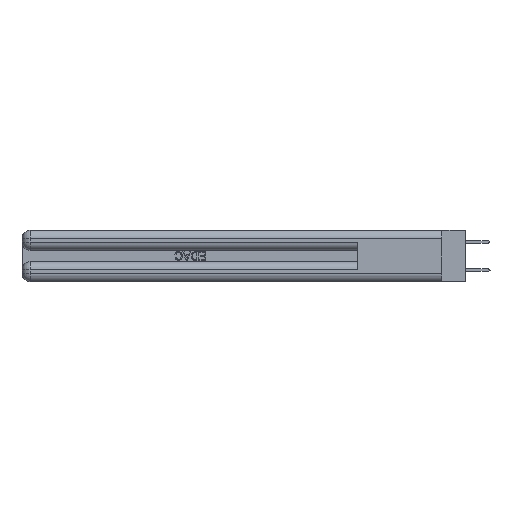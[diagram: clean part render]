
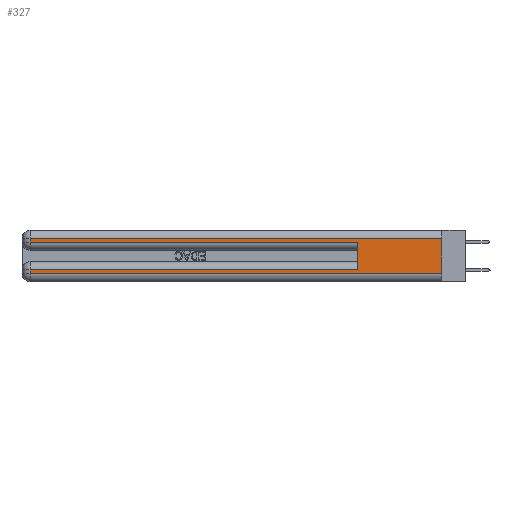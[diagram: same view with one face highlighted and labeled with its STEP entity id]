
A CAD part, left-side view. The second image highlights one B-rep face of the part: STEP entity #327.
In plain terms, the highlighted planar face has unit normal (-1, 0, 0).
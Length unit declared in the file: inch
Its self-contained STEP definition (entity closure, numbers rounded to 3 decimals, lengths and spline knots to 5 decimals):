
#327 = ADVANCED_FACE ( 'NONE', ( #8994 ), #20867, .F. ) ;
#1510 = LINE ( 'NONE', #37343, #40976 ) ;
#2214 = ORIENTED_EDGE ( 'NONE', *, *, #22925, .F. ) ;
#2718 = CARTESIAN_POINT ( 'NONE',  ( 0., 2.94, 0.37 ) ) ;
#3404 = ORIENTED_EDGE ( 'NONE', *, *, #18552, .T. ) ;
#4596 = DIRECTION ( 'NONE',  ( 0., -1., 0. ) ) ;
#6879 = DIRECTION ( 'NONE',  ( 0., 0., 1. ) ) ;
#6996 = ORIENTED_EDGE ( 'NONE', *, *, #29429, .T. ) ;
#7479 = VERTEX_POINT ( 'NONE', #31076 ) ;
#8994 = FACE_OUTER_BOUND ( 'NONE', #10043, .T. ) ;
#9367 = LINE ( 'NONE', #2718, #28560 ) ;
#9704 = CARTESIAN_POINT ( 'NONE',  ( 0., 0., 0.37 ) ) ;
#10043 = EDGE_LOOP ( 'NONE', ( #32769, #3404, #6996, #31560, #2214, #26198, #10621, #19074 ) ) ;
#10202 = DIRECTION ( 'NONE',  ( 0., 1., 0. ) ) ;
#10621 = ORIENTED_EDGE ( 'NONE', *, *, #47641, .T. ) ;
#10804 = VERTEX_POINT ( 'NONE', #34400 ) ;
#12850 = CARTESIAN_POINT ( 'NONE',  ( 0., 0., 0.31 ) ) ;
#14397 = CARTESIAN_POINT ( 'NONE',  ( 0., 2.94, 0.37 ) ) ;
#15383 = VECTOR ( 'NONE', #18261, 39.37008 ) ;
#16353 = VERTEX_POINT ( 'NONE', #48474 ) ;
#16963 = EDGE_CURVE ( 'NONE', #45041, #10804, #25833, .T. ) ;
#17001 = CARTESIAN_POINT ( 'NONE',  ( 0., 0., 0.37 ) ) ;
#17344 = LINE ( 'NONE', #9704, #27489 ) ;
#18261 = DIRECTION ( 'NONE',  ( 0., 0., -1. ) ) ;
#18550 = CARTESIAN_POINT ( 'NONE',  ( 0., 0.6, 0.285 ) ) ;
#18552 = EDGE_CURVE ( 'NONE', #7479, #30962, #46746, .T. ) ;
#18714 = CARTESIAN_POINT ( 'NONE',  ( 0., 2.94, 0.06 ) ) ;
#19074 = ORIENTED_EDGE ( 'NONE', *, *, #16963, .T. ) ;
#19959 = VERTEX_POINT ( 'NONE', #29063 ) ;
#20565 = DIRECTION ( 'NONE',  ( 0., 0., -1. ) ) ;
#20624 = VERTEX_POINT ( 'NONE', #18550 ) ;
#20867 = PLANE ( 'NONE',  #24140 ) ;
#22925 = EDGE_CURVE ( 'NONE', #34632, #20624, #1510, .T. ) ;
#24140 = AXIS2_PLACEMENT_3D ( 'NONE', #17001, #36191, #20565 ) ;
#25686 = DIRECTION ( 'NONE',  ( 0., 0., -1. ) ) ;
#25833 = LINE ( 'NONE', #33097, #44913 ) ;
#26198 = ORIENTED_EDGE ( 'NONE', *, *, #26421, .T. ) ;
#26421 = EDGE_CURVE ( 'NONE', #34632, #16353, #32372, .T. ) ;
#27489 = VECTOR ( 'NONE', #36467, 39.37008 ) ;
#28127 = EDGE_CURVE ( 'NONE', #7479, #10804, #17344, .T. ) ;
#28560 = VECTOR ( 'NONE', #25686, 39.37008 ) ;
#28891 = VECTOR ( 'NONE', #39566, 39.37008 ) ;
#29063 = CARTESIAN_POINT ( 'NONE',  ( 0., 2.94, 0.285 ) ) ;
#29429 = EDGE_CURVE ( 'NONE', #30962, #19959, #9367, .T. ) ;
#30962 = VERTEX_POINT ( 'NONE', #36897 ) ;
#31076 = CARTESIAN_POINT ( 'NONE',  ( 0., 0., 0.31 ) ) ;
#31153 = VECTOR ( 'NONE', #10202, 39.37008 ) ;
#31560 = ORIENTED_EDGE ( 'NONE', *, *, #47952, .T. ) ;
#32372 = LINE ( 'NONE', #33113, #31153 ) ;
#32699 = VECTOR ( 'NONE', #4596, 39.37008 ) ;
#32769 = ORIENTED_EDGE ( 'NONE', *, *, #28127, .F. ) ;
#33097 = CARTESIAN_POINT ( 'NONE',  ( 0., 0., 0.06 ) ) ;
#33113 = CARTESIAN_POINT ( 'NONE',  ( 0., 0., 0.085 ) ) ;
#34400 = CARTESIAN_POINT ( 'NONE',  ( 0., 0., 0.06 ) ) ;
#34632 = VERTEX_POINT ( 'NONE', #40692 ) ;
#36191 = DIRECTION ( 'NONE',  ( 1., 0., 0. ) ) ;
#36467 = DIRECTION ( 'NONE',  ( 0., 0., -1. ) ) ;
#36897 = CARTESIAN_POINT ( 'NONE',  ( 0., 2.94, 0.31 ) ) ;
#36920 = DIRECTION ( 'NONE',  ( 0., -1., 0. ) ) ;
#37343 = CARTESIAN_POINT ( 'NONE',  ( 0., 0.6, 0.145 ) ) ;
#39566 = DIRECTION ( 'NONE',  ( 0., 1., 0. ) ) ;
#40692 = CARTESIAN_POINT ( 'NONE',  ( 0., 0.6, 0.085 ) ) ;
#40976 = VECTOR ( 'NONE', #6879, 39.37008 ) ;
#42728 = CARTESIAN_POINT ( 'NONE',  ( 0., 0., 0.285 ) ) ;
#44019 = LINE ( 'NONE', #42728, #32699 ) ;
#44913 = VECTOR ( 'NONE', #36920, 39.37008 ) ;
#45041 = VERTEX_POINT ( 'NONE', #18714 ) ;
#45831 = LINE ( 'NONE', #14397, #15383 ) ;
#46746 = LINE ( 'NONE', #12850, #28891 ) ;
#47641 = EDGE_CURVE ( 'NONE', #16353, #45041, #45831, .T. ) ;
#47952 = EDGE_CURVE ( 'NONE', #19959, #20624, #44019, .T. ) ;
#48474 = CARTESIAN_POINT ( 'NONE',  ( 0., 2.94, 0.085 ) ) ;
